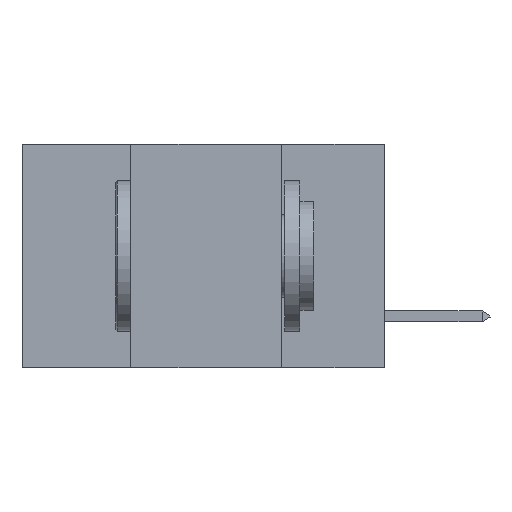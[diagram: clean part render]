
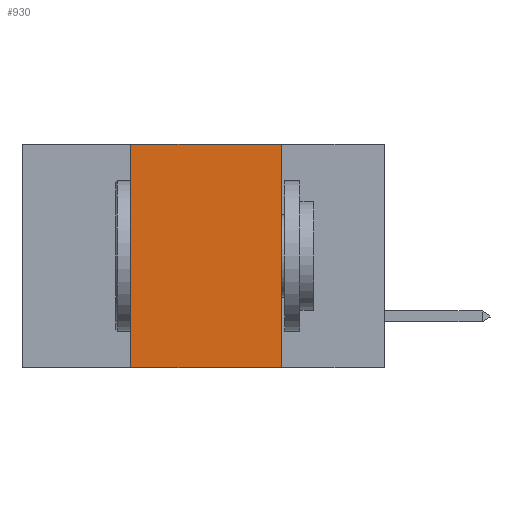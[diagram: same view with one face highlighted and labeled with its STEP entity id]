
A CAD part, left-side view. The second image highlights one B-rep face of the part: STEP entity #930.
In plain terms, the highlighted planar face has unit normal (-1, 0, 0).
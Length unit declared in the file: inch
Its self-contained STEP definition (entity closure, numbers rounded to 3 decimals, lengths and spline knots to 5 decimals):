
#930 = ADVANCED_FACE ( 'NONE', ( #22065 ), #36818, .F. ) ;
#3996 = DIRECTION ( 'NONE',  ( 0., 0., -1. ) ) ;
#5558 = VECTOR ( 'NONE', #34367, 39.37008 ) ;
#6157 = VECTOR ( 'NONE', #20190, 39.37008 ) ;
#6872 = CARTESIAN_POINT ( 'NONE',  ( 0., 0.6, -0.37 ) ) ;
#8939 = LINE ( 'NONE', #22906, #25240 ) ;
#10014 = LINE ( 'NONE', #6872, #19068 ) ;
#11079 = VERTEX_POINT ( 'NONE', #26774 ) ;
#11424 = EDGE_CURVE ( 'NONE', #11079, #21262, #10014, .T. ) ;
#13959 = VERTEX_POINT ( 'NONE', #35048 ) ;
#14978 = CARTESIAN_POINT ( 'NONE',  ( 0., 0.42, 0. ) ) ;
#15247 = CARTESIAN_POINT ( 'NONE',  ( 0., 0.6, 0. ) ) ;
#19068 = VECTOR ( 'NONE', #40349, 39.37008 ) ;
#19581 = ORIENTED_EDGE ( 'NONE', *, *, #37163, .F. ) ;
#19721 = ORIENTED_EDGE ( 'NONE', *, *, #11424, .T. ) ;
#20190 = DIRECTION ( 'NONE',  ( 0., -1., 0. ) ) ;
#21262 = VERTEX_POINT ( 'NONE', #23571 ) ;
#22065 = FACE_OUTER_BOUND ( 'NONE', #26694, .T. ) ;
#22213 = CARTESIAN_POINT ( 'NONE',  ( 0., 0.42, 0. ) ) ;
#22906 = CARTESIAN_POINT ( 'NONE',  ( 0., 0.17, 0. ) ) ;
#23290 = ORIENTED_EDGE ( 'NONE', *, *, #32402, .F. ) ;
#23571 = CARTESIAN_POINT ( 'NONE',  ( 0., 0.17, -0.37 ) ) ;
#24278 = LINE ( 'NONE', #14978, #5558 ) ;
#25240 = VECTOR ( 'NONE', #27281, 39.37008 ) ;
#26318 = VERTEX_POINT ( 'NONE', #22213 ) ;
#26694 = EDGE_LOOP ( 'NONE', ( #23290, #46426, #19581, #19721 ) ) ;
#26774 = CARTESIAN_POINT ( 'NONE',  ( 0., 0.42, -0.37 ) ) ;
#27212 = LINE ( 'NONE', #35504, #6157 ) ;
#27281 = DIRECTION ( 'NONE',  ( 0., 0., -1. ) ) ;
#28437 = AXIS2_PLACEMENT_3D ( 'NONE', #15247, #47681, #3996 ) ;
#32402 = EDGE_CURVE ( 'NONE', #13959, #21262, #8939, .T. ) ;
#34367 = DIRECTION ( 'NONE',  ( 0., 0., 1. ) ) ;
#35048 = CARTESIAN_POINT ( 'NONE',  ( 0., 0.17, 0. ) ) ;
#35504 = CARTESIAN_POINT ( 'NONE',  ( 0., 0.6, 0. ) ) ;
#36818 = PLANE ( 'NONE',  #28437 ) ;
#37163 = EDGE_CURVE ( 'NONE', #11079, #26318, #24278, .T. ) ;
#37484 = EDGE_CURVE ( 'NONE', #26318, #13959, #27212, .T. ) ;
#40349 = DIRECTION ( 'NONE',  ( 0., -1., 0. ) ) ;
#46426 = ORIENTED_EDGE ( 'NONE', *, *, #37484, .F. ) ;
#47681 = DIRECTION ( 'NONE',  ( 1., 0., 0. ) ) ;
